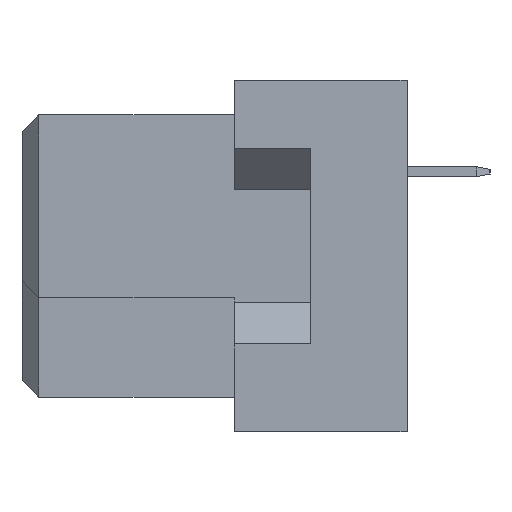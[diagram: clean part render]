
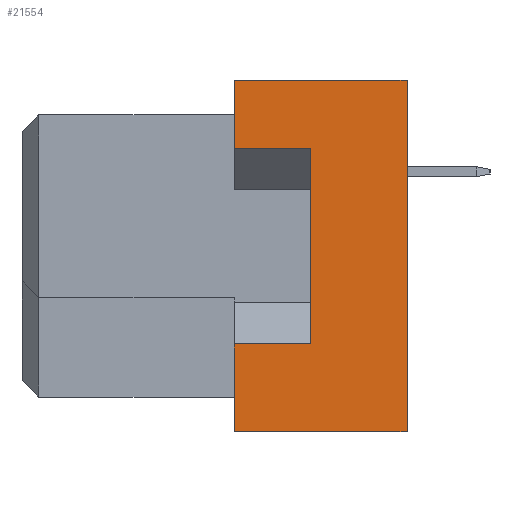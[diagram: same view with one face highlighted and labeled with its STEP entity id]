
A CAD part, left-side view. The second image highlights one B-rep face of the part: STEP entity #21554.
In plain terms, the highlighted planar face has unit normal (-1, 0, 0).
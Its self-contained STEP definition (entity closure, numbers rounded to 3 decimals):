
#151 = CARTESIAN_POINT ( 'NONE',  ( -47.5, -8.7, -2.65 ) ) ;
#1141 = LINE ( 'NONE', #22172, #27739 ) ;
#1459 = ORIENTED_EDGE ( 'NONE', *, *, #25970, .F. ) ;
#1808 = CARTESIAN_POINT ( 'NONE',  ( -47.5, -11.6, -5.3 ) ) ;
#2130 = CARTESIAN_POINT ( 'NONE',  ( -47.5, -8.7, 3.25 ) ) ;
#3331 = VERTEX_POINT ( 'NONE', #13451 ) ;
#3343 = ORIENTED_EDGE ( 'NONE', *, *, #9797, .T. ) ;
#4025 = EDGE_CURVE ( 'NONE', #27991, #3331, #10218, .T. ) ;
#4057 = VECTOR ( 'NONE', #24075, 1000. ) ;
#4065 = VERTEX_POINT ( 'NONE', #4799 ) ;
#4799 = CARTESIAN_POINT ( 'NONE',  ( -47.5, -6.4, 5.3 ) ) ;
#4918 = VERTEX_POINT ( 'NONE', #1808 ) ;
#5966 = PLANE ( 'NONE',  #30525 ) ;
#6149 = DIRECTION ( 'NONE',  ( -1., 0., 0. ) ) ;
#7061 = ORIENTED_EDGE ( 'NONE', *, *, #10140, .F. ) ;
#7824 = VERTEX_POINT ( 'NONE', #26082 ) ;
#7868 = ORIENTED_EDGE ( 'NONE', *, *, #10373, .F. ) ;
#8077 = EDGE_LOOP ( 'NONE', ( #29642, #27669, #1459, #22375, #3343, #7061, #17691, #7868 ) ) ;
#8290 = CARTESIAN_POINT ( 'NONE',  ( -47.5, -11.6, 5.3 ) ) ;
#9797 = EDGE_CURVE ( 'NONE', #12373, #4065, #16859, .T. ) ;
#10140 = EDGE_CURVE ( 'NONE', #7824, #4065, #28597, .T. ) ;
#10218 = LINE ( 'NONE', #19287, #16310 ) ;
#10373 = EDGE_CURVE ( 'NONE', #25613, #23220, #1141, .T. ) ;
#12373 = VERTEX_POINT ( 'NONE', #16119 ) ;
#12923 = DIRECTION ( 'NONE',  ( 0., 0., 1. ) ) ;
#13451 = CARTESIAN_POINT ( 'NONE',  ( -47.5, -6.4, -2.65 ) ) ;
#14020 = EDGE_CURVE ( 'NONE', #25613, #3331, #33360, .T. ) ;
#14528 = DIRECTION ( 'NONE',  ( 0., 1., 0. ) ) ;
#14640 = DIRECTION ( 'NONE',  ( 0., 1., 0. ) ) ;
#16119 = CARTESIAN_POINT ( 'NONE',  ( -47.5, -11.6, 5.3 ) ) ;
#16310 = VECTOR ( 'NONE', #19476, 1000. ) ;
#16859 = LINE ( 'NONE', #28645, #21650 ) ;
#17691 = ORIENTED_EDGE ( 'NONE', *, *, #37316, .F. ) ;
#19066 = DIRECTION ( 'NONE',  ( 0., 1., 0. ) ) ;
#19287 = CARTESIAN_POINT ( 'NONE',  ( -47.5, -6.4, -5.3 ) ) ;
#19476 = DIRECTION ( 'NONE',  ( 0., 0., 1. ) ) ;
#20438 = VECTOR ( 'NONE', #14640, 1000. ) ;
#20625 = FACE_OUTER_BOUND ( 'NONE', #8077, .T. ) ;
#21486 = VECTOR ( 'NONE', #19066, 1000. ) ;
#21554 = ADVANCED_FACE ( 'NONE', ( #20625 ), #5966, .T. ) ;
#21650 = VECTOR ( 'NONE', #14528, 1000. ) ;
#22172 = CARTESIAN_POINT ( 'NONE',  ( -47.5, -8.7, -2.65 ) ) ;
#22375 = ORIENTED_EDGE ( 'NONE', *, *, #33033, .T. ) ;
#22445 = LINE ( 'NONE', #34246, #33117 ) ;
#23220 = VERTEX_POINT ( 'NONE', #2130 ) ;
#24075 = DIRECTION ( 'NONE',  ( 0., 1., 0. ) ) ;
#25613 = VERTEX_POINT ( 'NONE', #151 ) ;
#25970 = EDGE_CURVE ( 'NONE', #4918, #27991, #34324, .T. ) ;
#26075 = DIRECTION ( 'NONE',  ( 0., 0., 1. ) ) ;
#26082 = CARTESIAN_POINT ( 'NONE',  ( -47.5, -6.4, 3.25 ) ) ;
#26977 = LINE ( 'NONE', #29513, #20438 ) ;
#27548 = CARTESIAN_POINT ( 'NONE',  ( -47.5, -8.7, -2.65 ) ) ;
#27669 = ORIENTED_EDGE ( 'NONE', *, *, #4025, .F. ) ;
#27739 = VECTOR ( 'NONE', #12923, 1000. ) ;
#27991 = VERTEX_POINT ( 'NONE', #37139 ) ;
#28597 = LINE ( 'NONE', #28979, #30293 ) ;
#28645 = CARTESIAN_POINT ( 'NONE',  ( -47.5, -11.6, 5.3 ) ) ;
#28979 = CARTESIAN_POINT ( 'NONE',  ( -47.5, -6.4, -5.3 ) ) ;
#29513 = CARTESIAN_POINT ( 'NONE',  ( -47.5, -8.7, 3.25 ) ) ;
#29642 = ORIENTED_EDGE ( 'NONE', *, *, #14020, .T. ) ;
#29723 = DIRECTION ( 'NONE',  ( 0., 0., 1. ) ) ;
#30293 = VECTOR ( 'NONE', #26075, 1000. ) ;
#30525 = AXIS2_PLACEMENT_3D ( 'NONE', #8290, #6149, #29723 ) ;
#33033 = EDGE_CURVE ( 'NONE', #4918, #12373, #22445, .T. ) ;
#33117 = VECTOR ( 'NONE', #34433, 1000. ) ;
#33360 = LINE ( 'NONE', #27548, #4057 ) ;
#34246 = CARTESIAN_POINT ( 'NONE',  ( -47.5, -11.6, 5.3 ) ) ;
#34324 = LINE ( 'NONE', #36649, #21486 ) ;
#34433 = DIRECTION ( 'NONE',  ( 0., 0., 1. ) ) ;
#36649 = CARTESIAN_POINT ( 'NONE',  ( -47.5, -11.6, -5.3 ) ) ;
#37139 = CARTESIAN_POINT ( 'NONE',  ( -47.5, -6.4, -5.3 ) ) ;
#37316 = EDGE_CURVE ( 'NONE', #23220, #7824, #26977, .T. ) ;
